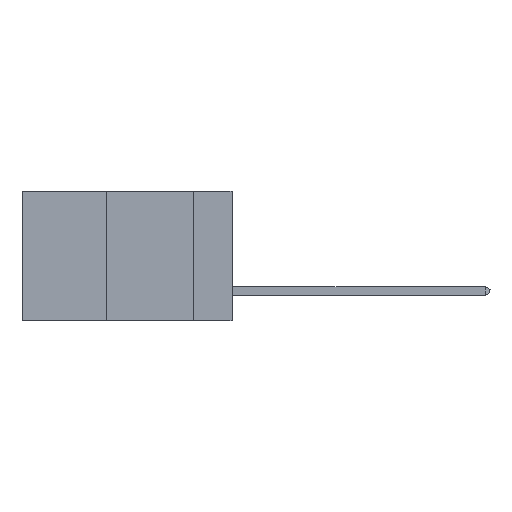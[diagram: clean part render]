
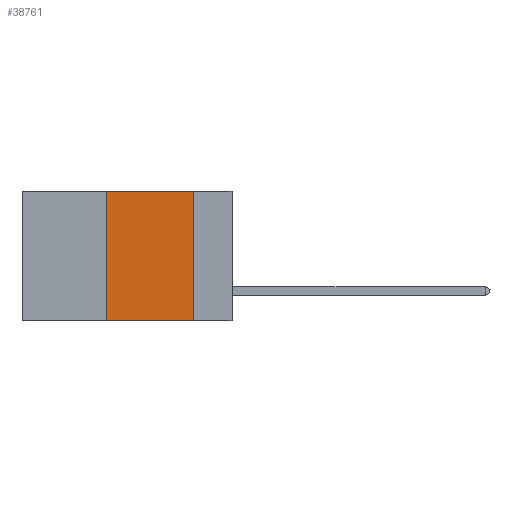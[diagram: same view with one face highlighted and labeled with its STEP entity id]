
A CAD part, left-side view. The second image highlights one B-rep face of the part: STEP entity #38761.
In plain terms, the highlighted planar face has unit normal (-1, 0, 0).
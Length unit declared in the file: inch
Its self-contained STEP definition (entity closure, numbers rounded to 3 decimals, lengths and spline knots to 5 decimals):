
#518 = CARTESIAN_POINT ( 'NONE',  ( 0., 0.6, -0.37 ) ) ;
#855 = CARTESIAN_POINT ( 'NONE',  ( 0., 0.36, 0. ) ) ;
#1000 = AXIS2_PLACEMENT_3D ( 'NONE', #2638, #2360, #24885 ) ;
#2166 = VECTOR ( 'NONE', #29674, 39.37008 ) ;
#2360 = DIRECTION ( 'NONE',  ( 1., 0., 0. ) ) ;
#2638 = CARTESIAN_POINT ( 'NONE',  ( 0., 0.6, 0. ) ) ;
#3287 = DIRECTION ( 'NONE',  ( 0., 0., -1. ) ) ;
#3690 = DIRECTION ( 'NONE',  ( 0., -1., 0. ) ) ;
#3857 = CARTESIAN_POINT ( 'NONE',  ( 0., 0.11, 0. ) ) ;
#4757 = FACE_OUTER_BOUND ( 'NONE', #28321, .T. ) ;
#4868 = VERTEX_POINT ( 'NONE', #3857 ) ;
#7186 = LINE ( 'NONE', #518, #2166 ) ;
#7188 = CARTESIAN_POINT ( 'NONE',  ( 0., 0.6, 0. ) ) ;
#8010 = EDGE_CURVE ( 'NONE', #4868, #28940, #14136, .T. ) ;
#14136 = LINE ( 'NONE', #16488, #20571 ) ;
#16488 = CARTESIAN_POINT ( 'NONE',  ( 0., 0.11, 0. ) ) ;
#16974 = ORIENTED_EDGE ( 'NONE', *, *, #23966, .T. ) ;
#20172 = LINE ( 'NONE', #7188, #27678 ) ;
#20571 = VECTOR ( 'NONE', #3287, 39.37008 ) ;
#22188 = VECTOR ( 'NONE', #39955, 39.37008 ) ;
#23966 = EDGE_CURVE ( 'NONE', #34382, #28940, #7186, .T. ) ;
#24584 = PLANE ( 'NONE',  #1000 ) ;
#24885 = DIRECTION ( 'NONE',  ( 0., 0., -1. ) ) ;
#26617 = CARTESIAN_POINT ( 'NONE',  ( 0., 0.36, 0. ) ) ;
#27678 = VECTOR ( 'NONE', #3690, 39.37008 ) ;
#28321 = EDGE_LOOP ( 'NONE', ( #31309, #33505, #35079, #16974 ) ) ;
#28940 = VERTEX_POINT ( 'NONE', #36763 ) ;
#29674 = DIRECTION ( 'NONE',  ( 0., -1., 0. ) ) ;
#31139 = EDGE_CURVE ( 'NONE', #37804, #4868, #20172, .T. ) ;
#31309 = ORIENTED_EDGE ( 'NONE', *, *, #8010, .F. ) ;
#33350 = CARTESIAN_POINT ( 'NONE',  ( 0., 0.36, -0.37 ) ) ;
#33505 = ORIENTED_EDGE ( 'NONE', *, *, #31139, .F. ) ;
#34240 = LINE ( 'NONE', #26617, #22188 ) ;
#34382 = VERTEX_POINT ( 'NONE', #33350 ) ;
#35079 = ORIENTED_EDGE ( 'NONE', *, *, #37947, .F. ) ;
#36763 = CARTESIAN_POINT ( 'NONE',  ( 0., 0.11, -0.37 ) ) ;
#37804 = VERTEX_POINT ( 'NONE', #855 ) ;
#37947 = EDGE_CURVE ( 'NONE', #34382, #37804, #34240, .T. ) ;
#38761 = ADVANCED_FACE ( 'NONE', ( #4757 ), #24584, .F. ) ;
#39955 = DIRECTION ( 'NONE',  ( 0., 0., 1. ) ) ;
